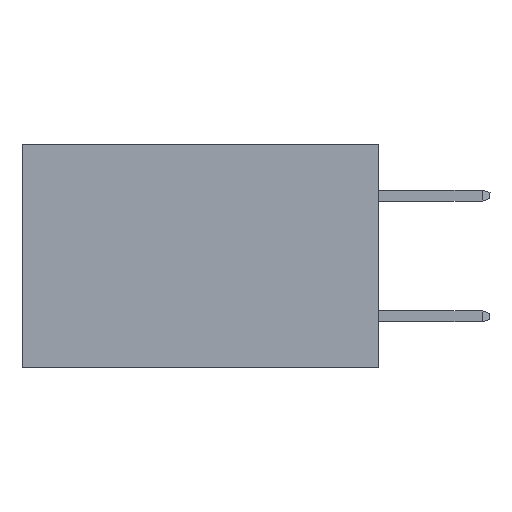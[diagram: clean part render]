
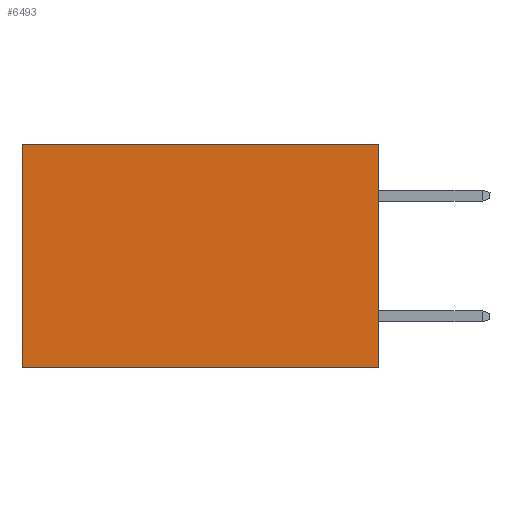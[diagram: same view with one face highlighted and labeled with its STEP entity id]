
A CAD part, left-side view. The second image highlights one B-rep face of the part: STEP entity #6493.
In plain terms, the highlighted planar face has unit normal (-1, 0, 0).
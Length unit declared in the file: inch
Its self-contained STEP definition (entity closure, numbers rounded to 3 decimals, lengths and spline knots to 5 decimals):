
#76 = EDGE_CURVE ( 'NONE', #6618, #2418, #6802, .T. ) ;
#149 = ORIENTED_EDGE ( 'NONE', *, *, #4325, .T. ) ;
#234 = FACE_OUTER_BOUND ( 'NONE', #8783, .T. ) ;
#941 = CARTESIAN_POINT ( 'NONE',  ( 0.277, 0., 0. ) ) ;
#1237 = ORIENTED_EDGE ( 'NONE', *, *, #8446, .F. ) ;
#1427 = ORIENTED_EDGE ( 'NONE', *, *, #7054, .F. ) ;
#1706 = LINE ( 'NONE', #8185, #3543 ) ;
#1722 = CARTESIAN_POINT ( 'NONE',  ( 0.277, 0., -0.37 ) ) ;
#2105 = ORIENTED_EDGE ( 'NONE', *, *, #76, .T. ) ;
#2302 = AXIS2_PLACEMENT_3D ( 'NONE', #3328, #3394, #3178 ) ;
#2418 = VERTEX_POINT ( 'NONE', #3586 ) ;
#2505 = CARTESIAN_POINT ( 'NONE',  ( 0.277, 0., 0. ) ) ;
#3178 = DIRECTION ( 'NONE',  ( 0., 0., -1. ) ) ;
#3261 = PLANE ( 'NONE',  #2302 ) ;
#3328 = CARTESIAN_POINT ( 'NONE',  ( 0.277, 0., -0.37 ) ) ;
#3394 = DIRECTION ( 'NONE',  ( 1., 0., 0. ) ) ;
#3449 = CARTESIAN_POINT ( 'NONE',  ( 0.277, 0.59, -0.37 ) ) ;
#3543 = VECTOR ( 'NONE', #8878, 39.37008 ) ;
#3586 = CARTESIAN_POINT ( 'NONE',  ( 0.277, 0.59, 0. ) ) ;
#3839 = DIRECTION ( 'NONE',  ( 0., 0., -1. ) ) ;
#4325 = EDGE_CURVE ( 'NONE', #2418, #7876, #9619, .T. ) ;
#4415 = VECTOR ( 'NONE', #6803, 39.37008 ) ;
#5230 = VERTEX_POINT ( 'NONE', #7987 ) ;
#6360 = CARTESIAN_POINT ( 'NONE',  ( 0.277, 0.59, -0.37 ) ) ;
#6493 = ADVANCED_FACE ( 'NONE', ( #234 ), #3261, .F. ) ;
#6618 = VERTEX_POINT ( 'NONE', #941 ) ;
#6802 = LINE ( 'NONE', #2505, #4415 ) ;
#6803 = DIRECTION ( 'NONE',  ( 0., 1., 0. ) ) ;
#7054 = EDGE_CURVE ( 'NONE', #6618, #5230, #9330, .T. ) ;
#7520 = VECTOR ( 'NONE', #9214, 39.37008 ) ;
#7846 = VECTOR ( 'NONE', #3839, 39.37008 ) ;
#7876 = VERTEX_POINT ( 'NONE', #6360 ) ;
#7987 = CARTESIAN_POINT ( 'NONE',  ( 0.277, 0., -0.37 ) ) ;
#8185 = CARTESIAN_POINT ( 'NONE',  ( 0.277, 0., -0.37 ) ) ;
#8446 = EDGE_CURVE ( 'NONE', #5230, #7876, #1706, .T. ) ;
#8783 = EDGE_LOOP ( 'NONE', ( #149, #1237, #1427, #2105 ) ) ;
#8878 = DIRECTION ( 'NONE',  ( 0., 1., 0. ) ) ;
#9214 = DIRECTION ( 'NONE',  ( 0., 0., -1. ) ) ;
#9330 = LINE ( 'NONE', #1722, #7520 ) ;
#9619 = LINE ( 'NONE', #3449, #7846 ) ;
